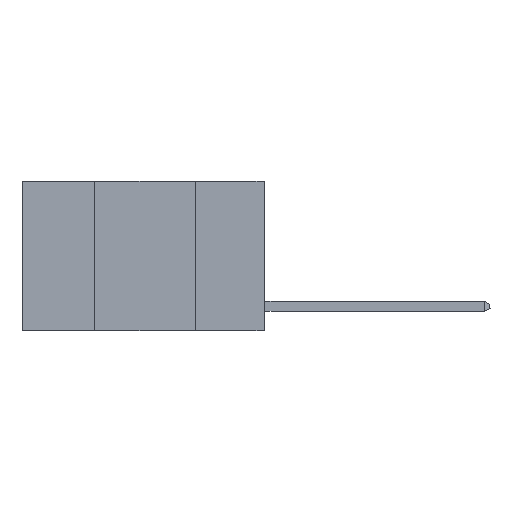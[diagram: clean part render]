
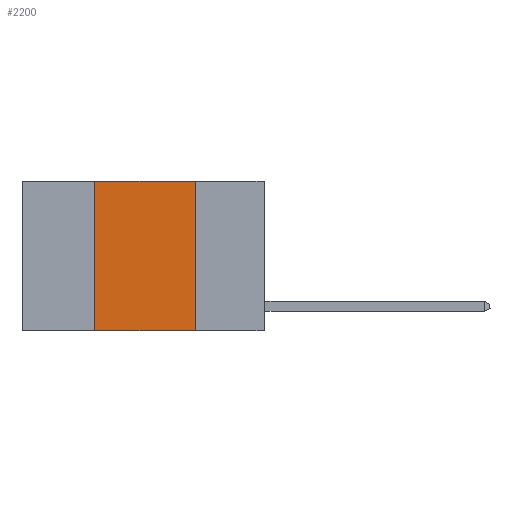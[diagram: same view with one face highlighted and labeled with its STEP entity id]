
A CAD part, left-side view. The second image highlights one B-rep face of the part: STEP entity #2200.
In plain terms, the highlighted planar face has unit normal (-1, 0, 0).
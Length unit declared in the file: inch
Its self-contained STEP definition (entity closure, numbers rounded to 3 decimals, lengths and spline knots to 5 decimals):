
#823 = VERTEX_POINT ( 'NONE', #13343 ) ;
#1046 = CARTESIAN_POINT ( 'NONE',  ( 0., 0.6, -0.37 ) ) ;
#2200 = ADVANCED_FACE ( 'NONE', ( #8221 ), #16049, .F. ) ;
#2553 = VECTOR ( 'NONE', #3174, 39.37008 ) ;
#2559 = VECTOR ( 'NONE', #21795, 39.37008 ) ;
#2668 = ORIENTED_EDGE ( 'NONE', *, *, #6611, .F. ) ;
#3114 = DIRECTION ( 'NONE',  ( 0., 0., 1. ) ) ;
#3174 = DIRECTION ( 'NONE',  ( 0., 0., -1. ) ) ;
#3696 = AXIS2_PLACEMENT_3D ( 'NONE', #14120, #11930, #19759 ) ;
#4102 = CARTESIAN_POINT ( 'NONE',  ( 0., 0.17, 0. ) ) ;
#4735 = VECTOR ( 'NONE', #12615, 39.37008 ) ;
#4833 = VERTEX_POINT ( 'NONE', #4102 ) ;
#5276 = ORIENTED_EDGE ( 'NONE', *, *, #11917, .T. ) ;
#6611 = EDGE_CURVE ( 'NONE', #7064, #4833, #11680, .T. ) ;
#7064 = VERTEX_POINT ( 'NONE', #7558 ) ;
#7558 = CARTESIAN_POINT ( 'NONE',  ( 0., 0.42, 0. ) ) ;
#8221 = FACE_OUTER_BOUND ( 'NONE', #8474, .T. ) ;
#8474 = EDGE_LOOP ( 'NONE', ( #21560, #2668, #21638, #5276 ) ) ;
#9155 = LINE ( 'NONE', #13014, #2553 ) ;
#11680 = LINE ( 'NONE', #19508, #2559 ) ;
#11917 = EDGE_CURVE ( 'NONE', #823, #13030, #18648, .T. ) ;
#11930 = DIRECTION ( 'NONE',  ( 1., 0., 0. ) ) ;
#12615 = DIRECTION ( 'NONE',  ( 0., -1., 0. ) ) ;
#13014 = CARTESIAN_POINT ( 'NONE',  ( 0., 0.17, 0. ) ) ;
#13030 = VERTEX_POINT ( 'NONE', #14060 ) ;
#13343 = CARTESIAN_POINT ( 'NONE',  ( 0., 0.42, -0.37 ) ) ;
#14060 = CARTESIAN_POINT ( 'NONE',  ( 0., 0.17, -0.37 ) ) ;
#14120 = CARTESIAN_POINT ( 'NONE',  ( 0., 0.6, 0. ) ) ;
#15472 = VECTOR ( 'NONE', #3114, 39.37008 ) ;
#16049 = PLANE ( 'NONE',  #3696 ) ;
#18648 = LINE ( 'NONE', #1046, #4735 ) ;
#19508 = CARTESIAN_POINT ( 'NONE',  ( 0., 0.6, 0. ) ) ;
#19759 = DIRECTION ( 'NONE',  ( 0., 0., -1. ) ) ;
#21560 = ORIENTED_EDGE ( 'NONE', *, *, #22542, .F. ) ;
#21638 = ORIENTED_EDGE ( 'NONE', *, *, #24884, .F. ) ;
#21795 = DIRECTION ( 'NONE',  ( 0., -1., 0. ) ) ;
#22285 = CARTESIAN_POINT ( 'NONE',  ( 0., 0.42, 0. ) ) ;
#22542 = EDGE_CURVE ( 'NONE', #4833, #13030, #9155, .T. ) ;
#24436 = LINE ( 'NONE', #22285, #15472 ) ;
#24884 = EDGE_CURVE ( 'NONE', #823, #7064, #24436, .T. ) ;
